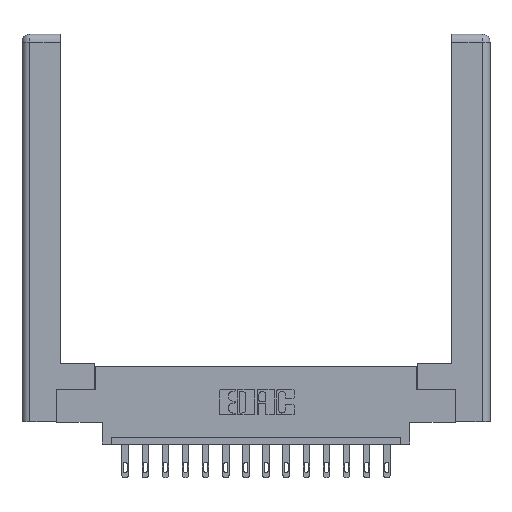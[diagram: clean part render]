
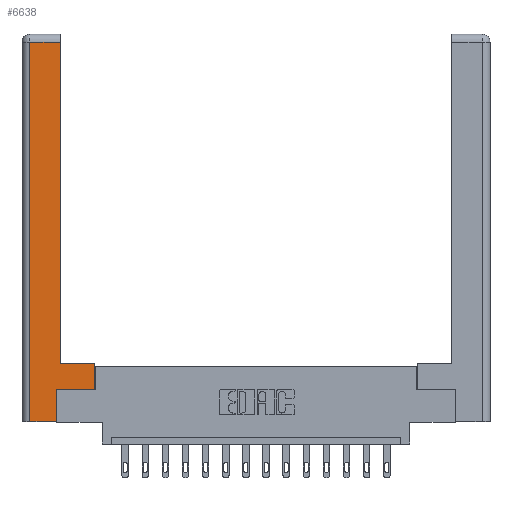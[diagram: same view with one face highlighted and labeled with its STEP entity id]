
A CAD part, top view. The second image highlights one B-rep face of the part: STEP entity #6638.
In plain terms, the highlighted planar face has unit normal (0, 0, 1).
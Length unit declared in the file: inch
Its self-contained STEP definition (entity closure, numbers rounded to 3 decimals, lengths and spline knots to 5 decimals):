
#608 = PLANE ( 'NONE',  #3148 ) ;
#615 = CARTESIAN_POINT ( 'NONE',  ( 0.295, 3., 0. ) ) ;
#1298 = VERTEX_POINT ( 'NONE', #12014 ) ;
#1803 = CARTESIAN_POINT ( 'NONE',  ( 0.295, 2.94, 0. ) ) ;
#1941 = DIRECTION ( 'NONE',  ( 0., 0., -1. ) ) ;
#2236 = DIRECTION ( 'NONE',  ( -1., 0., 0. ) ) ;
#2431 = LINE ( 'NONE', #10803, #13127 ) ;
#2620 = CARTESIAN_POINT ( 'NONE',  ( 0.565, 0.245, 0. ) ) ;
#3148 = AXIS2_PLACEMENT_3D ( 'NONE', #14726, #1941, #10965 ) ;
#3471 = CARTESIAN_POINT ( 'NONE',  ( 0.0615, 2.94, 0. ) ) ;
#3472 = DIRECTION ( 'NONE',  ( -1., 0., 0. ) ) ;
#3710 = LINE ( 'NONE', #3471, #13004 ) ;
#3784 = CARTESIAN_POINT ( 'NONE',  ( 0.0615, 2.94, 0. ) ) ;
#3871 = VECTOR ( 'NONE', #3472, 39.37008 ) ;
#3907 = DIRECTION ( 'NONE',  ( 0., 1., 0. ) ) ;
#4213 = LINE ( 'NONE', #5081, #9052 ) ;
#4371 = EDGE_CURVE ( 'NONE', #1298, #6795, #8787, .T. ) ;
#4839 = ORIENTED_EDGE ( 'NONE', *, *, #11196, .T. ) ;
#4984 = CARTESIAN_POINT ( 'NONE',  ( 0.265, 0.245, 0. ) ) ;
#5081 = CARTESIAN_POINT ( 'NONE',  ( 0.565, 0.245, 0. ) ) ;
#5556 = VECTOR ( 'NONE', #13555, 39.37008 ) ;
#6274 = CARTESIAN_POINT ( 'NONE',  ( 0.565, 0.45, 0. ) ) ;
#6334 = DIRECTION ( 'NONE',  ( 1., 0., 0. ) ) ;
#6410 = VECTOR ( 'NONE', #9430, 39.37008 ) ;
#6617 = ORIENTED_EDGE ( 'NONE', *, *, #9494, .T. ) ;
#6638 = ADVANCED_FACE ( 'NONE', ( #8804 ), #608, .F. ) ;
#6795 = VERTEX_POINT ( 'NONE', #1803 ) ;
#6820 = LINE ( 'NONE', #12262, #6410 ) ;
#6824 = ORIENTED_EDGE ( 'NONE', *, *, #15849, .T. ) ;
#6880 = DIRECTION ( 'NONE',  ( 0., -1., 0. ) ) ;
#7288 = VERTEX_POINT ( 'NONE', #14564 ) ;
#7589 = ORIENTED_EDGE ( 'NONE', *, *, #9938, .T. ) ;
#7621 = VERTEX_POINT ( 'NONE', #3784 ) ;
#7899 = EDGE_CURVE ( 'NONE', #6795, #7621, #3710, .T. ) ;
#7914 = LINE ( 'NONE', #8609, #3871 ) ;
#8154 = VERTEX_POINT ( 'NONE', #4984 ) ;
#8566 = ORIENTED_EDGE ( 'NONE', *, *, #7899, .T. ) ;
#8609 = CARTESIAN_POINT ( 'NONE',  ( 0.295, 0.45, 0. ) ) ;
#8708 = VERTEX_POINT ( 'NONE', #12078 ) ;
#8785 = LINE ( 'NONE', #14552, #9015 ) ;
#8787 = LINE ( 'NONE', #615, #5556 ) ;
#8804 = FACE_OUTER_BOUND ( 'NONE', #10485, .T. ) ;
#9015 = VECTOR ( 'NONE', #6880, 39.37008 ) ;
#9024 = EDGE_CURVE ( 'NONE', #13569, #7288, #11765, .T. ) ;
#9052 = VECTOR ( 'NONE', #6334, 39.37008 ) ;
#9324 = VECTOR ( 'NONE', #3907, 39.37008 ) ;
#9430 = DIRECTION ( 'NONE',  ( 1., 0., 0. ) ) ;
#9494 = EDGE_CURVE ( 'NONE', #7288, #1298, #7914, .T. ) ;
#9938 = EDGE_CURVE ( 'NONE', #8708, #8154, #2431, .T. ) ;
#10485 = EDGE_LOOP ( 'NONE', ( #10845, #8566, #11925, #6824, #7589, #4839, #15531, #6617 ) ) ;
#10803 = CARTESIAN_POINT ( 'NONE',  ( 0.265, 0.245, 0. ) ) ;
#10845 = ORIENTED_EDGE ( 'NONE', *, *, #4371, .T. ) ;
#10965 = DIRECTION ( 'NONE',  ( -1., 0., 0. ) ) ;
#11196 = EDGE_CURVE ( 'NONE', #8154, #13569, #4213, .T. ) ;
#11765 = LINE ( 'NONE', #6274, #9324 ) ;
#11925 = ORIENTED_EDGE ( 'NONE', *, *, #15825, .T. ) ;
#12014 = CARTESIAN_POINT ( 'NONE',  ( 0.295, 0.45, 0. ) ) ;
#12078 = CARTESIAN_POINT ( 'NONE',  ( 0.265, 0., 0. ) ) ;
#12110 = DIRECTION ( 'NONE',  ( 0., 1., 0. ) ) ;
#12262 = CARTESIAN_POINT ( 'NONE',  ( 0.265, 0., 0. ) ) ;
#12817 = CARTESIAN_POINT ( 'NONE',  ( 0.0615, 0., 0. ) ) ;
#13004 = VECTOR ( 'NONE', #2236, 39.37008 ) ;
#13127 = VECTOR ( 'NONE', #12110, 39.37008 ) ;
#13555 = DIRECTION ( 'NONE',  ( 0., 1., 0. ) ) ;
#13569 = VERTEX_POINT ( 'NONE', #2620 ) ;
#14552 = CARTESIAN_POINT ( 'NONE',  ( 0.0615, 0., 0. ) ) ;
#14564 = CARTESIAN_POINT ( 'NONE',  ( 0.565, 0.45, 0. ) ) ;
#14726 = CARTESIAN_POINT ( 'NONE',  ( 0., 0., 0. ) ) ;
#14943 = VERTEX_POINT ( 'NONE', #12817 ) ;
#15531 = ORIENTED_EDGE ( 'NONE', *, *, #9024, .T. ) ;
#15825 = EDGE_CURVE ( 'NONE', #7621, #14943, #8785, .T. ) ;
#15849 = EDGE_CURVE ( 'NONE', #14943, #8708, #6820, .T. ) ;
